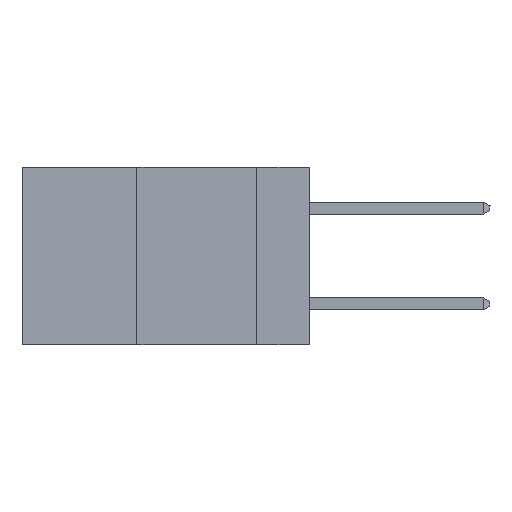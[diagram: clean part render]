
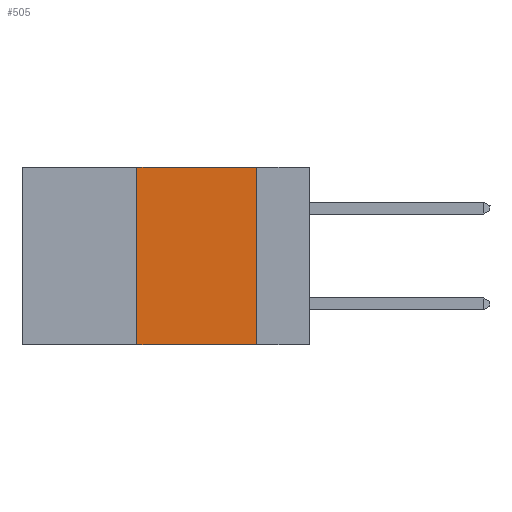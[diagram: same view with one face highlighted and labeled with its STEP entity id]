
A CAD part, left-side view. The second image highlights one B-rep face of the part: STEP entity #505.
In plain terms, the highlighted planar face has unit normal (-1, 0, 0).
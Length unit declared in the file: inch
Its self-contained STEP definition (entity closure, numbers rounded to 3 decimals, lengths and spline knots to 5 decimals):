
#224 = EDGE_CURVE ( 'NONE', #3214, #6053, #13662, .T. ) ;
#293 = VERTEX_POINT ( 'NONE', #13514 ) ;
#453 = CARTESIAN_POINT ( 'NONE',  ( 0., 0.11, -0.37 ) ) ;
#505 = ADVANCED_FACE ( 'NONE', ( #12100 ), #5070, .F. ) ;
#595 = DIRECTION ( 'NONE',  ( 0., 0., -1. ) ) ;
#897 = CARTESIAN_POINT ( 'NONE',  ( 0., 0.36, 0. ) ) ;
#1461 = EDGE_LOOP ( 'NONE', ( #4840, #12420, #12364, #14369 ) ) ;
#2104 = LINE ( 'NONE', #2928, #10550 ) ;
#2609 = CARTESIAN_POINT ( 'NONE',  ( 0., 0.36, 0. ) ) ;
#2928 = CARTESIAN_POINT ( 'NONE',  ( 0., 0.11, 0. ) ) ;
#3214 = VERTEX_POINT ( 'NONE', #8200 ) ;
#4836 = VERTEX_POINT ( 'NONE', #2609 ) ;
#4840 = ORIENTED_EDGE ( 'NONE', *, *, #13554, .F. ) ;
#5070 = PLANE ( 'NONE',  #11855 ) ;
#5090 = VECTOR ( 'NONE', #9024, 39.37008 ) ;
#5616 = CARTESIAN_POINT ( 'NONE',  ( 0., 0.6, 0. ) ) ;
#6053 = VERTEX_POINT ( 'NONE', #453 ) ;
#7563 = VECTOR ( 'NONE', #8642, 39.37008 ) ;
#8080 = EDGE_CURVE ( 'NONE', #3214, #4836, #14248, .T. ) ;
#8200 = CARTESIAN_POINT ( 'NONE',  ( 0., 0.36, -0.37 ) ) ;
#8642 = DIRECTION ( 'NONE',  ( 0., 0., 1. ) ) ;
#8850 = EDGE_CURVE ( 'NONE', #4836, #293, #10003, .T. ) ;
#8964 = DIRECTION ( 'NONE',  ( 0., -1., 0. ) ) ;
#9024 = DIRECTION ( 'NONE',  ( 0., -1., 0. ) ) ;
#10003 = LINE ( 'NONE', #5616, #12055 ) ;
#10550 = VECTOR ( 'NONE', #11966, 39.37008 ) ;
#11855 = AXIS2_PLACEMENT_3D ( 'NONE', #12030, #14406, #595 ) ;
#11966 = DIRECTION ( 'NONE',  ( 0., 0., -1. ) ) ;
#12030 = CARTESIAN_POINT ( 'NONE',  ( 0., 0.6, 0. ) ) ;
#12055 = VECTOR ( 'NONE', #8964, 39.37008 ) ;
#12100 = FACE_OUTER_BOUND ( 'NONE', #1461, .T. ) ;
#12364 = ORIENTED_EDGE ( 'NONE', *, *, #8080, .F. ) ;
#12420 = ORIENTED_EDGE ( 'NONE', *, *, #8850, .F. ) ;
#13514 = CARTESIAN_POINT ( 'NONE',  ( 0., 0.11, 0. ) ) ;
#13554 = EDGE_CURVE ( 'NONE', #293, #6053, #2104, .T. ) ;
#13662 = LINE ( 'NONE', #14569, #5090 ) ;
#14248 = LINE ( 'NONE', #897, #7563 ) ;
#14369 = ORIENTED_EDGE ( 'NONE', *, *, #224, .T. ) ;
#14406 = DIRECTION ( 'NONE',  ( 1., 0., 0. ) ) ;
#14569 = CARTESIAN_POINT ( 'NONE',  ( 0., 0.6, -0.37 ) ) ;
